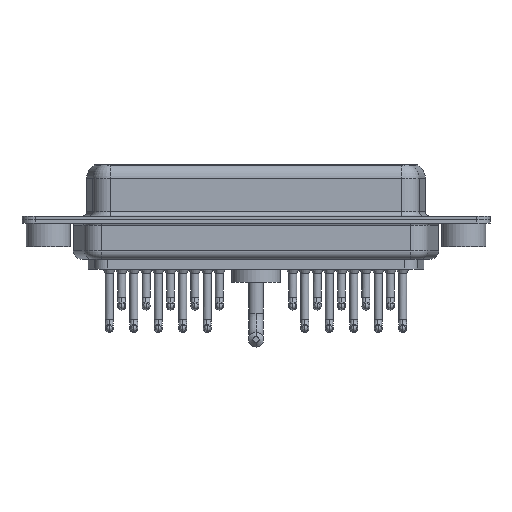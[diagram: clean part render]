
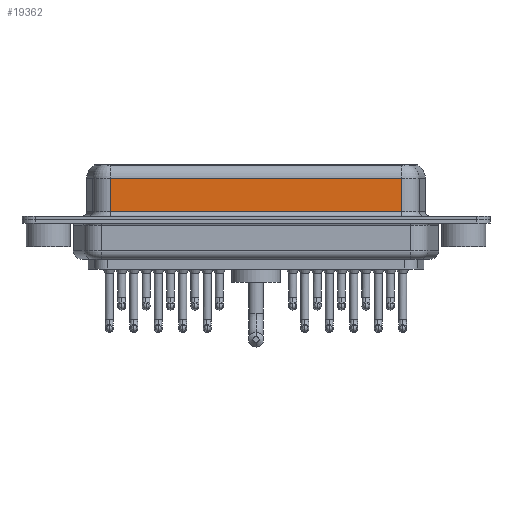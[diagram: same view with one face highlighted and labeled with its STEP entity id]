
A CAD part, front view. The second image highlights one B-rep face of the part: STEP entity #19362.
In plain terms, the highlighted planar face has unit normal (0, -1, 0).
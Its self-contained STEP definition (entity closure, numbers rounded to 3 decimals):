
#103 = DIRECTION ( 'NONE',  ( 0., 1., 0. ) ) ;
#762 = EDGE_LOOP ( 'NONE', ( #18768, #926, #16615, #8736 ) ) ;
#841 = DIRECTION ( 'NONE',  ( 0., 0., -1. ) ) ;
#926 = ORIENTED_EDGE ( 'NONE', *, *, #18802, .T. ) ;
#2261 = VERTEX_POINT ( 'NONE', #6312 ) ;
#4087 = LINE ( 'NONE', #19905, #8010 ) ;
#6312 = CARTESIAN_POINT ( 'NONE',  ( 40.037, -3.95, 4.65 ) ) ;
#7224 = CARTESIAN_POINT ( 'NONE',  ( 40.037, -3.95, 6.4 ) ) ;
#7229 = CARTESIAN_POINT ( 'NONE',  ( 40.037, -3.95, 0.9 ) ) ;
#7458 = PLANE ( 'NONE',  #17505 ) ;
#7748 = DIRECTION ( 'NONE',  ( 0., 0., -1. ) ) ;
#8010 = VECTOR ( 'NONE', #7748, 1000. ) ;
#8196 = CARTESIAN_POINT ( 'NONE',  ( 7.013, -3.95, 4.65 ) ) ;
#8289 = VECTOR ( 'NONE', #19294, 1000. ) ;
#8736 = ORIENTED_EDGE ( 'NONE', *, *, #19773, .T. ) ;
#8789 = VERTEX_POINT ( 'NONE', #20933 ) ;
#10466 = LINE ( 'NONE', #11966, #8289 ) ;
#11486 = VERTEX_POINT ( 'NONE', #8196 ) ;
#11629 = LINE ( 'NONE', #16556, #15477 ) ;
#11966 = CARTESIAN_POINT ( 'NONE',  ( 40.037, -3.95, 4.65 ) ) ;
#12239 = VERTEX_POINT ( 'NONE', #7229 ) ;
#12682 = LINE ( 'NONE', #21735, #17157 ) ;
#13503 = EDGE_CURVE ( 'NONE', #11486, #8789, #11629, .T. ) ;
#15477 = VECTOR ( 'NONE', #841, 1000. ) ;
#16556 = CARTESIAN_POINT ( 'NONE',  ( 7.013, -3.95, 6.4 ) ) ;
#16615 = ORIENTED_EDGE ( 'NONE', *, *, #13503, .T. ) ;
#17157 = VECTOR ( 'NONE', #17840, 1000. ) ;
#17505 = AXIS2_PLACEMENT_3D ( 'NONE', #7224, #103, #21557 ) ;
#17782 = FACE_OUTER_BOUND ( 'NONE', #762, .T. ) ;
#17840 = DIRECTION ( 'NONE',  ( 1., 0., 0. ) ) ;
#18768 = ORIENTED_EDGE ( 'NONE', *, *, #19882, .F. ) ;
#18802 = EDGE_CURVE ( 'NONE', #2261, #11486, #10466, .T. ) ;
#19294 = DIRECTION ( 'NONE',  ( -1., 0., 0. ) ) ;
#19362 = ADVANCED_FACE ( 'NONE', ( #17782 ), #7458, .F. ) ;
#19773 = EDGE_CURVE ( 'NONE', #8789, #12239, #12682, .T. ) ;
#19882 = EDGE_CURVE ( 'NONE', #2261, #12239, #4087, .T. ) ;
#19905 = CARTESIAN_POINT ( 'NONE',  ( 40.037, -3.95, 6.4 ) ) ;
#20933 = CARTESIAN_POINT ( 'NONE',  ( 7.013, -3.95, 0.9 ) ) ;
#21557 = DIRECTION ( 'NONE',  ( 0., 0., 1. ) ) ;
#21735 = CARTESIAN_POINT ( 'NONE',  ( 40.037, -3.95, 0.9 ) ) ;
